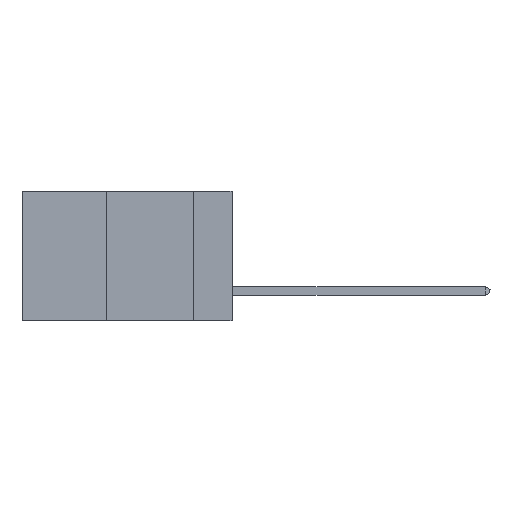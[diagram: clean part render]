
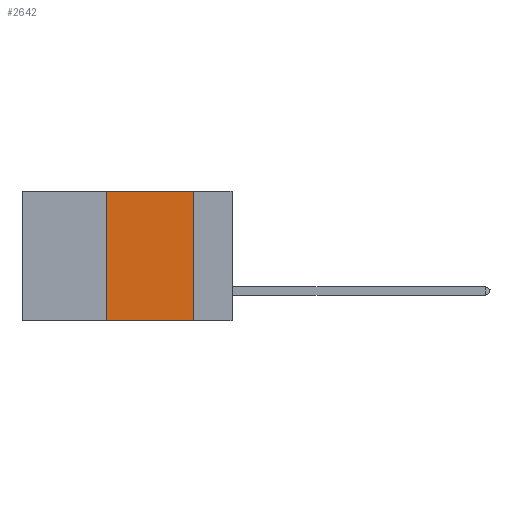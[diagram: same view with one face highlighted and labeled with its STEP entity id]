
A CAD part, left-side view. The second image highlights one B-rep face of the part: STEP entity #2642.
In plain terms, the highlighted planar face has unit normal (-1, 0, 0).
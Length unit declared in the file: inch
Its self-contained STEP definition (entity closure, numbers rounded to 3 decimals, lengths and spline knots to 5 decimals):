
#455 = LINE ( 'NONE', #21962, #14138 ) ;
#704 = DIRECTION ( 'NONE',  ( 0., -1., 0. ) ) ;
#1551 = PLANE ( 'NONE',  #32182 ) ;
#2031 = VERTEX_POINT ( 'NONE', #34108 ) ;
#2642 = ADVANCED_FACE ( 'NONE', ( #28442 ), #1551, .F. ) ;
#4378 = EDGE_CURVE ( 'NONE', #26355, #37127, #455, .T. ) ;
#5228 = EDGE_LOOP ( 'NONE', ( #26964, #27240, #32400, #34532 ) ) ;
#6064 = VECTOR ( 'NONE', #27086, 39.37008 ) ;
#6161 = VECTOR ( 'NONE', #32839, 39.37008 ) ;
#7763 = CARTESIAN_POINT ( 'NONE',  ( 0., 0.6, 0. ) ) ;
#8013 = CARTESIAN_POINT ( 'NONE',  ( 0., 0.36, 0. ) ) ;
#10049 = VECTOR ( 'NONE', #28011, 39.37008 ) ;
#11305 = VERTEX_POINT ( 'NONE', #19113 ) ;
#12000 = CARTESIAN_POINT ( 'NONE',  ( 0., 0.6, -0.37 ) ) ;
#14138 = VECTOR ( 'NONE', #704, 39.37008 ) ;
#15016 = CARTESIAN_POINT ( 'NONE',  ( 0., 0.11, 0. ) ) ;
#16711 = LINE ( 'NONE', #12000, #10049 ) ;
#19113 = CARTESIAN_POINT ( 'NONE',  ( 0., 0.11, -0.37 ) ) ;
#20966 = EDGE_CURVE ( 'NONE', #37127, #11305, #25986, .T. ) ;
#21498 = CARTESIAN_POINT ( 'NONE',  ( 0., 0.36, 0. ) ) ;
#21962 = CARTESIAN_POINT ( 'NONE',  ( 0., 0.6, 0. ) ) ;
#24346 = EDGE_CURVE ( 'NONE', #2031, #11305, #16711, .T. ) ;
#25986 = LINE ( 'NONE', #15016, #6161 ) ;
#26355 = VERTEX_POINT ( 'NONE', #8013 ) ;
#26964 = ORIENTED_EDGE ( 'NONE', *, *, #20966, .F. ) ;
#27086 = DIRECTION ( 'NONE',  ( 0., 0., 1. ) ) ;
#27240 = ORIENTED_EDGE ( 'NONE', *, *, #4378, .F. ) ;
#28011 = DIRECTION ( 'NONE',  ( 0., -1., 0. ) ) ;
#28442 = FACE_OUTER_BOUND ( 'NONE', #5228, .T. ) ;
#28639 = DIRECTION ( 'NONE',  ( 1., 0., 0. ) ) ;
#32182 = AXIS2_PLACEMENT_3D ( 'NONE', #7763, #28639, #37751 ) ;
#32400 = ORIENTED_EDGE ( 'NONE', *, *, #37041, .F. ) ;
#32839 = DIRECTION ( 'NONE',  ( 0., 0., -1. ) ) ;
#33812 = CARTESIAN_POINT ( 'NONE',  ( 0., 0.11, 0. ) ) ;
#34108 = CARTESIAN_POINT ( 'NONE',  ( 0., 0.36, -0.37 ) ) ;
#34532 = ORIENTED_EDGE ( 'NONE', *, *, #24346, .T. ) ;
#37041 = EDGE_CURVE ( 'NONE', #2031, #26355, #38677, .T. ) ;
#37127 = VERTEX_POINT ( 'NONE', #33812 ) ;
#37751 = DIRECTION ( 'NONE',  ( 0., 0., -1. ) ) ;
#38677 = LINE ( 'NONE', #21498, #6064 ) ;
